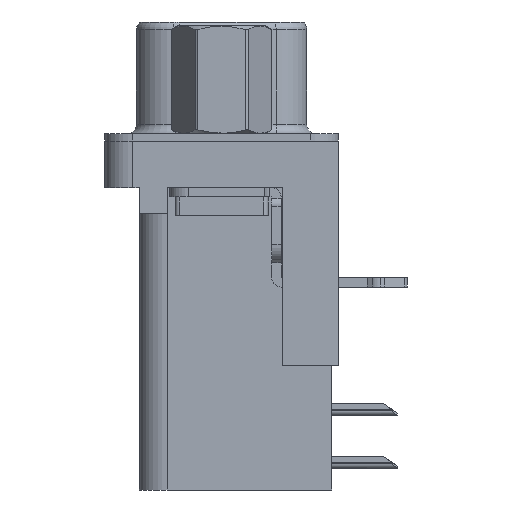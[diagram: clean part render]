
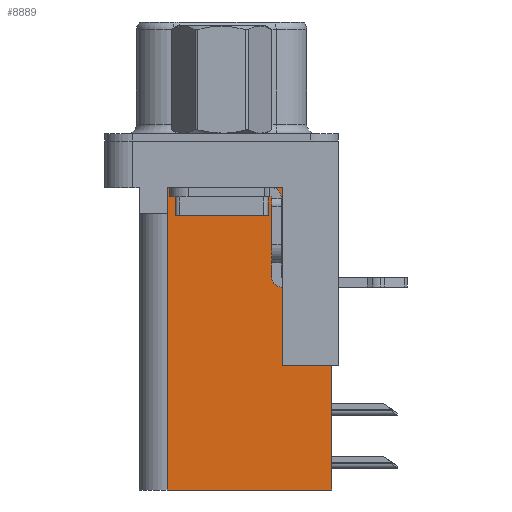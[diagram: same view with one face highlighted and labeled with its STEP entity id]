
A CAD part, left-side view. The second image highlights one B-rep face of the part: STEP entity #8889.
In plain terms, the highlighted planar face has unit normal (-1, 0, 0).
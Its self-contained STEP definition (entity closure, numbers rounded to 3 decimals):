
#131 = CARTESIAN_POINT ( 'NONE',  ( 3.7, 2.895, -3.9 ) ) ;
#1113 = CARTESIAN_POINT ( 'NONE',  ( 3.7, -3.295, -2.5 ) ) ;
#1432 = VERTEX_POINT ( 'NONE', #4703 ) ;
#2577 = VERTEX_POINT ( 'NONE', #22105 ) ;
#2782 = DIRECTION ( 'NONE',  ( 0., 1., 0. ) ) ;
#3286 = CARTESIAN_POINT ( 'NONE',  ( 3.7, 0., -3.9 ) ) ;
#4116 = EDGE_CURVE ( 'NONE', #4160, #26144, #12150, .T. ) ;
#4150 = FACE_OUTER_BOUND ( 'NONE', #7767, .T. ) ;
#4160 = VERTEX_POINT ( 'NONE', #131 ) ;
#4703 = CARTESIAN_POINT ( 'NONE',  ( 3.7, -5.925, -18.76 ) ) ;
#4880 = VECTOR ( 'NONE', #14122, 1000. ) ;
#5237 = VECTOR ( 'NONE', #7285, 1000. ) ;
#5258 = CARTESIAN_POINT ( 'NONE',  ( 3.7, -3.295, -18.76 ) ) ;
#5383 = EDGE_CURVE ( 'NONE', #23986, #1432, #9065, .T. ) ;
#5405 = LINE ( 'NONE', #5258, #11128 ) ;
#5681 = ORIENTED_EDGE ( 'NONE', *, *, #11149, .F. ) ;
#5797 = VERTEX_POINT ( 'NONE', #23519 ) ;
#6981 = LINE ( 'NONE', #25501, #23687 ) ;
#7258 = ORIENTED_EDGE ( 'NONE', *, *, #19407, .T. ) ;
#7285 = DIRECTION ( 'NONE',  ( 0., 1., 0. ) ) ;
#7767 = EDGE_LOOP ( 'NONE', ( #7258, #17136, #17769, #27213, #5681, #9368, #8025, #21811 ) ) ;
#8025 = ORIENTED_EDGE ( 'NONE', *, *, #27846, .T. ) ;
#8391 = VECTOR ( 'NONE', #28060, 1000. ) ;
#8889 = ADVANCED_FACE ( 'NONE', ( #4150 ), #27063, .F. ) ;
#9065 = LINE ( 'NONE', #23965, #8391 ) ;
#9368 = ORIENTED_EDGE ( 'NONE', *, *, #5383, .F. ) ;
#9669 = DIRECTION ( 'NONE',  ( 1., 0., 0. ) ) ;
#9865 = EDGE_CURVE ( 'NONE', #15836, #26144, #21480, .T. ) ;
#10215 = CARTESIAN_POINT ( 'NONE',  ( 3.7, -3.295, -12.05 ) ) ;
#10778 = CARTESIAN_POINT ( 'NONE',  ( 3.7, -3.295, -18.76 ) ) ;
#10790 = LINE ( 'NONE', #10778, #15953 ) ;
#11128 = VECTOR ( 'NONE', #14012, 1000. ) ;
#11149 = EDGE_CURVE ( 'NONE', #1432, #15836, #10790, .T. ) ;
#11428 = VECTOR ( 'NONE', #2782, 1000. ) ;
#11944 = CARTESIAN_POINT ( 'NONE',  ( 3.7, -5.925, -12.05 ) ) ;
#12150 = LINE ( 'NONE', #3286, #11428 ) ;
#13537 = CARTESIAN_POINT ( 'NONE',  ( 3.7, 2.925, -18.76 ) ) ;
#13953 = EDGE_CURVE ( 'NONE', #5797, #4160, #6981, .T. ) ;
#14012 = DIRECTION ( 'NONE',  ( 0., 0., 1. ) ) ;
#14122 = DIRECTION ( 'NONE',  ( 0., 1., 0. ) ) ;
#14622 = DIRECTION ( 'NONE',  ( 0., 0., -1. ) ) ;
#15217 = DIRECTION ( 'NONE',  ( 0., 1., 0. ) ) ;
#15543 = CARTESIAN_POINT ( 'NONE',  ( 3.7, 2.925, -18.76 ) ) ;
#15652 = DIRECTION ( 'NONE',  ( 0., 0., 1. ) ) ;
#15836 = VERTEX_POINT ( 'NONE', #15543 ) ;
#15953 = VECTOR ( 'NONE', #15217, 1000. ) ;
#17136 = ORIENTED_EDGE ( 'NONE', *, *, #13953, .T. ) ;
#17769 = ORIENTED_EDGE ( 'NONE', *, *, #4116, .T. ) ;
#18080 = AXIS2_PLACEMENT_3D ( 'NONE', #22726, #9669, #24965 ) ;
#18828 = VERTEX_POINT ( 'NONE', #10215 ) ;
#19407 = EDGE_CURVE ( 'NONE', #2577, #5797, #21568, .T. ) ;
#20340 = CARTESIAN_POINT ( 'NONE',  ( 3.7, -6.295, -12.05 ) ) ;
#20585 = LINE ( 'NONE', #20340, #5237 ) ;
#21480 = LINE ( 'NONE', #13537, #25940 ) ;
#21568 = LINE ( 'NONE', #1113, #4880 ) ;
#21811 = ORIENTED_EDGE ( 'NONE', *, *, #23453, .T. ) ;
#22105 = CARTESIAN_POINT ( 'NONE',  ( 3.7, -3.295, -2.5 ) ) ;
#22726 = CARTESIAN_POINT ( 'NONE',  ( 3.7, -3.295, -18.76 ) ) ;
#23453 = EDGE_CURVE ( 'NONE', #18828, #2577, #5405, .T. ) ;
#23519 = CARTESIAN_POINT ( 'NONE',  ( 3.7, 2.895, -2.5 ) ) ;
#23687 = VECTOR ( 'NONE', #14622, 1000. ) ;
#23965 = CARTESIAN_POINT ( 'NONE',  ( 3.7, -5.925, -2. ) ) ;
#23986 = VERTEX_POINT ( 'NONE', #11944 ) ;
#24965 = DIRECTION ( 'NONE',  ( 0., 1., 0. ) ) ;
#25501 = CARTESIAN_POINT ( 'NONE',  ( 3.7, 2.895, -3.9 ) ) ;
#25940 = VECTOR ( 'NONE', #15652, 1000. ) ;
#26144 = VERTEX_POINT ( 'NONE', #27809 ) ;
#27063 = PLANE ( 'NONE',  #18080 ) ;
#27213 = ORIENTED_EDGE ( 'NONE', *, *, #9865, .F. ) ;
#27809 = CARTESIAN_POINT ( 'NONE',  ( 3.7, 2.925, -3.9 ) ) ;
#27846 = EDGE_CURVE ( 'NONE', #23986, #18828, #20585, .T. ) ;
#28060 = DIRECTION ( 'NONE',  ( 0., 0., -1. ) ) ;
